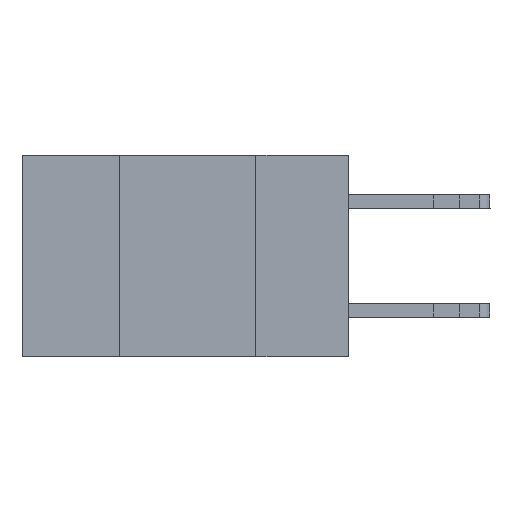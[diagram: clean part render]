
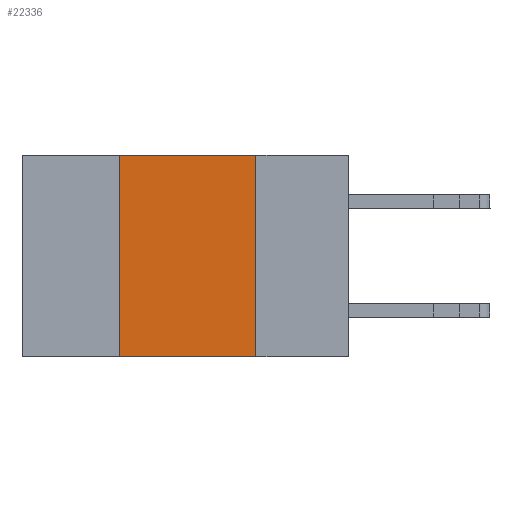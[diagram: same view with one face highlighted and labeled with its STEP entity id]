
A CAD part, left-side view. The second image highlights one B-rep face of the part: STEP entity #22336.
In plain terms, the highlighted planar face has unit normal (-1, 0, 0).
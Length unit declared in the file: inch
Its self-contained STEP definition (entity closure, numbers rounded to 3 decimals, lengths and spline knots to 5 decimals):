
#1553 = PLANE ( 'NONE',  #11968 ) ;
#2886 = LINE ( 'NONE', #22074, #12033 ) ;
#3110 = EDGE_CURVE ( 'NONE', #17015, #14079, #7609, .T. ) ;
#4333 = EDGE_CURVE ( 'NONE', #15837, #17015, #6433, .T. ) ;
#5231 = DIRECTION ( 'NONE',  ( 1., 0., 0. ) ) ;
#5900 = VECTOR ( 'NONE', #22121, 39.37008 ) ;
#6396 = CARTESIAN_POINT ( 'NONE',  ( 0., 0.6, 0. ) ) ;
#6433 = LINE ( 'NONE', #11107, #20390 ) ;
#6490 = DIRECTION ( 'NONE',  ( 0., -1., 0. ) ) ;
#7609 = LINE ( 'NONE', #6396, #10483 ) ;
#9206 = ORIENTED_EDGE ( 'NONE', *, *, #20682, .F. ) ;
#9372 = CARTESIAN_POINT ( 'NONE',  ( 0., 0.42, 0. ) ) ;
#10483 = VECTOR ( 'NONE', #6490, 39.37008 ) ;
#11103 = DIRECTION ( 'NONE',  ( 0., 0., 1. ) ) ;
#11107 = CARTESIAN_POINT ( 'NONE',  ( 0., 0.42, -0.37 ) ) ;
#11166 = CARTESIAN_POINT ( 'NONE',  ( 0., 0.6, -0.37 ) ) ;
#11968 = AXIS2_PLACEMENT_3D ( 'NONE', #16130, #5231, #18013 ) ;
#12019 = CARTESIAN_POINT ( 'NONE',  ( 0., 0.42, -0.37 ) ) ;
#12033 = VECTOR ( 'NONE', #14674, 39.37008 ) ;
#12889 = EDGE_CURVE ( 'NONE', #15837, #21074, #14993, .T. ) ;
#14079 = VERTEX_POINT ( 'NONE', #19749 ) ;
#14674 = DIRECTION ( 'NONE',  ( 0., 0., -1. ) ) ;
#14993 = LINE ( 'NONE', #11166, #5900 ) ;
#15837 = VERTEX_POINT ( 'NONE', #12019 ) ;
#15908 = FACE_OUTER_BOUND ( 'NONE', #20979, .T. ) ;
#15993 = ORIENTED_EDGE ( 'NONE', *, *, #12889, .T. ) ;
#16130 = CARTESIAN_POINT ( 'NONE',  ( 0., 0.6, 0. ) ) ;
#17015 = VERTEX_POINT ( 'NONE', #9372 ) ;
#18013 = DIRECTION ( 'NONE',  ( 0., 0., -1. ) ) ;
#19144 = ORIENTED_EDGE ( 'NONE', *, *, #3110, .F. ) ;
#19749 = CARTESIAN_POINT ( 'NONE',  ( 0., 0.17, 0. ) ) ;
#20390 = VECTOR ( 'NONE', #11103, 39.37008 ) ;
#20682 = EDGE_CURVE ( 'NONE', #14079, #21074, #2886, .T. ) ;
#20979 = EDGE_LOOP ( 'NONE', ( #9206, #19144, #21185, #15993 ) ) ;
#21074 = VERTEX_POINT ( 'NONE', #23092 ) ;
#21185 = ORIENTED_EDGE ( 'NONE', *, *, #4333, .F. ) ;
#22074 = CARTESIAN_POINT ( 'NONE',  ( 0., 0.17, -0.37 ) ) ;
#22121 = DIRECTION ( 'NONE',  ( 0., -1., 0. ) ) ;
#22336 = ADVANCED_FACE ( 'NONE', ( #15908 ), #1553, .F. ) ;
#23092 = CARTESIAN_POINT ( 'NONE',  ( 0., 0.17, -0.37 ) ) ;
